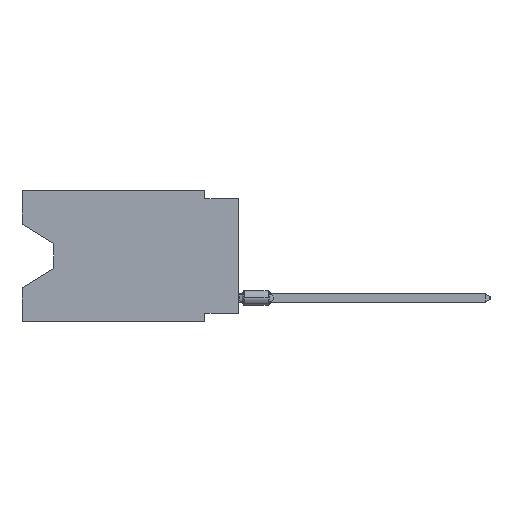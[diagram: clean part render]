
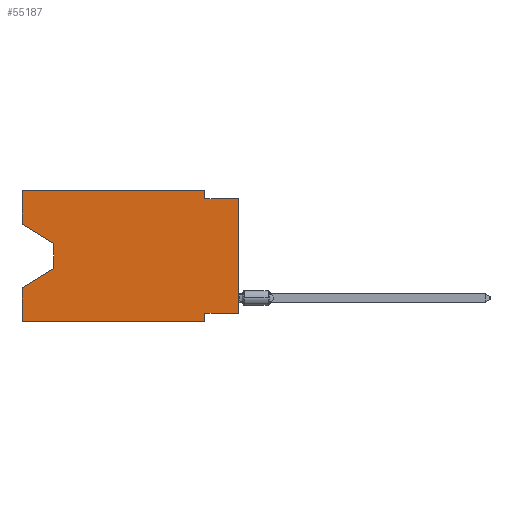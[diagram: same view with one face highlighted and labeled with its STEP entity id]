
A CAD part, left-side view. The second image highlights one B-rep face of the part: STEP entity #55187.
In plain terms, the highlighted planar face has unit normal (-1, 0, 0).
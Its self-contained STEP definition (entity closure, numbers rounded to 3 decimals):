
#244 = LINE ( 'NONE', #58147, #23302 ) ;
#911 = VERTEX_POINT ( 'NONE', #13001 ) ;
#1676 = EDGE_CURVE ( 'NONE', #24414, #61593, #34540, .T. ) ;
#2221 = DIRECTION ( 'NONE',  ( 0., -1., 0. ) ) ;
#2526 = VECTOR ( 'NONE', #54785, 1000. ) ;
#3853 = VECTOR ( 'NONE', #38729, 1000. ) ;
#5923 = CARTESIAN_POINT ( 'NONE',  ( 0., 16.383, 0. ) ) ;
#5988 = LINE ( 'NONE', #9868, #21817 ) ;
#6323 = DIRECTION ( 'NONE',  ( 0., 0., -1. ) ) ;
#6400 = AXIS2_PLACEMENT_3D ( 'NONE', #39036, #55075, #6996 ) ;
#6870 = CARTESIAN_POINT ( 'NONE',  ( 0., 0., -0.635 ) ) ;
#6996 = DIRECTION ( 'NONE',  ( 0., 0., -1. ) ) ;
#7610 = CARTESIAN_POINT ( 'NONE',  ( 0., 2.54, -9.271 ) ) ;
#7929 = CARTESIAN_POINT ( 'NONE',  ( 0., 16.383, -7.36 ) ) ;
#8169 = CARTESIAN_POINT ( 'NONE',  ( 0., 0., -0.635 ) ) ;
#9366 = ORIENTED_EDGE ( 'NONE', *, *, #19558, .F. ) ;
#9517 = VECTOR ( 'NONE', #2221, 1000. ) ;
#9868 = CARTESIAN_POINT ( 'NONE',  ( 0., 2.54, -9.906 ) ) ;
#10898 = VERTEX_POINT ( 'NONE', #7929 ) ;
#11689 = VERTEX_POINT ( 'NONE', #51573 ) ;
#12729 = VECTOR ( 'NONE', #14229, 1000. ) ;
#13001 = CARTESIAN_POINT ( 'NONE',  ( 0., 2.54, -9.906 ) ) ;
#13111 = CARTESIAN_POINT ( 'NONE',  ( 0., 0., -9.271 ) ) ;
#13189 = LINE ( 'NONE', #13889, #12729 ) ;
#13889 = CARTESIAN_POINT ( 'NONE',  ( 0., 16.383, 0. ) ) ;
#14229 = DIRECTION ( 'NONE',  ( 0., 0., 1. ) ) ;
#14278 = VECTOR ( 'NONE', #56601, 1000. ) ;
#15689 = DIRECTION ( 'NONE',  ( 0., -1., 0. ) ) ;
#16171 = VERTEX_POINT ( 'NONE', #47012 ) ;
#18167 = CARTESIAN_POINT ( 'NONE',  ( 0., 16.383, 0. ) ) ;
#19558 = EDGE_CURVE ( 'NONE', #32609, #10898, #38389, .T. ) ;
#19913 = ORIENTED_EDGE ( 'NONE', *, *, #37666, .T. ) ;
#20381 = EDGE_CURVE ( 'NONE', #32609, #911, #60815, .T. ) ;
#21331 = DIRECTION ( 'NONE',  ( 0., -0.855, -0.519 ) ) ;
#21817 = VECTOR ( 'NONE', #31117, 1000. ) ;
#22386 = LINE ( 'NONE', #64577, #2526 ) ;
#22391 = CARTESIAN_POINT ( 'NONE',  ( 0., 13.97, -4.013 ) ) ;
#23302 = VECTOR ( 'NONE', #53229, 1000. ) ;
#23369 = CARTESIAN_POINT ( 'NONE',  ( 0., 13.97, -5.893 ) ) ;
#24414 = VERTEX_POINT ( 'NONE', #49823 ) ;
#24623 = EDGE_CURVE ( 'NONE', #60272, #49423, #244, .T. ) ;
#24779 = DIRECTION ( 'NONE',  ( 0., 0., 1. ) ) ;
#27459 = ORIENTED_EDGE ( 'NONE', *, *, #1676, .F. ) ;
#27554 = FACE_OUTER_BOUND ( 'NONE', #32052, .T. ) ;
#28298 = VECTOR ( 'NONE', #15689, 1000. ) ;
#28327 = EDGE_CURVE ( 'NONE', #11689, #24414, #57886, .T. ) ;
#28705 = CARTESIAN_POINT ( 'NONE',  ( 0., 16.383, -9.906 ) ) ;
#29189 = VECTOR ( 'NONE', #21331, 1000. ) ;
#31117 = DIRECTION ( 'NONE',  ( 0., 0., -1. ) ) ;
#31757 = VERTEX_POINT ( 'NONE', #6870 ) ;
#32052 = EDGE_LOOP ( 'NONE', ( #51289, #41936, #38336, #9366, #62065, #38538, #60744, #19913, #34408, #27459, #47963, #59722 ) ) ;
#32609 = VERTEX_POINT ( 'NONE', #28705 ) ;
#32967 = EDGE_CURVE ( 'NONE', #49884, #911, #5988, .T. ) ;
#34408 = ORIENTED_EDGE ( 'NONE', *, *, #42374, .F. ) ;
#34540 = LINE ( 'NONE', #54399, #65931 ) ;
#37359 = LINE ( 'NONE', #37703, #29189 ) ;
#37666 = EDGE_CURVE ( 'NONE', #59210, #31757, #51957, .T. ) ;
#37703 = CARTESIAN_POINT ( 'NONE',  ( 0., 16.383, -2.546 ) ) ;
#38336 = ORIENTED_EDGE ( 'NONE', *, *, #62720, .T. ) ;
#38389 = LINE ( 'NONE', #18167, #3853 ) ;
#38538 = ORIENTED_EDGE ( 'NONE', *, *, #32967, .F. ) ;
#38729 = DIRECTION ( 'NONE',  ( 0., 0., 1. ) ) ;
#39036 = CARTESIAN_POINT ( 'NONE',  ( 0., 16.383, 0. ) ) ;
#40620 = EDGE_CURVE ( 'NONE', #59210, #49884, #65741, .T. ) ;
#41936 = ORIENTED_EDGE ( 'NONE', *, *, #24623, .T. ) ;
#42374 = EDGE_CURVE ( 'NONE', #61593, #31757, #61506, .T. ) ;
#43424 = DIRECTION ( 'NONE',  ( 0., 1., 0. ) ) ;
#45515 = VECTOR ( 'NONE', #24779, 1000. ) ;
#47012 = CARTESIAN_POINT ( 'NONE',  ( 0., 16.383, -2.546 ) ) ;
#47412 = EDGE_CURVE ( 'NONE', #16171, #60272, #37359, .T. ) ;
#47963 = ORIENTED_EDGE ( 'NONE', *, *, #28327, .F. ) ;
#48800 = PLANE ( 'NONE',  #6400 ) ;
#49017 = CARTESIAN_POINT ( 'NONE',  ( 0., 0., -9.271 ) ) ;
#49423 = VERTEX_POINT ( 'NONE', #23369 ) ;
#49624 = CARTESIAN_POINT ( 'NONE',  ( 0., 16.383, -9.906 ) ) ;
#49823 = CARTESIAN_POINT ( 'NONE',  ( 0., 2.54, 0. ) ) ;
#49884 = VERTEX_POINT ( 'NONE', #7610 ) ;
#51289 = ORIENTED_EDGE ( 'NONE', *, *, #47412, .T. ) ;
#51573 = CARTESIAN_POINT ( 'NONE',  ( 0., 16.383, 0. ) ) ;
#51607 = CARTESIAN_POINT ( 'NONE',  ( 0., 0., 0. ) ) ;
#51700 = EDGE_CURVE ( 'NONE', #16171, #11689, #13189, .T. ) ;
#51957 = LINE ( 'NONE', #51607, #45515 ) ;
#53229 = DIRECTION ( 'NONE',  ( 0., 0., -1. ) ) ;
#54399 = CARTESIAN_POINT ( 'NONE',  ( 0., 2.54, 0. ) ) ;
#54785 = DIRECTION ( 'NONE',  ( 0., 0.855, -0.519 ) ) ;
#55075 = DIRECTION ( 'NONE',  ( 1., 0., 0. ) ) ;
#55187 = ADVANCED_FACE ( 'NONE', ( #27554 ), #48800, .F. ) ;
#56601 = DIRECTION ( 'NONE',  ( 0., -1., 0. ) ) ;
#57886 = LINE ( 'NONE', #5923, #28298 ) ;
#58147 = CARTESIAN_POINT ( 'NONE',  ( 0., 13.97, -4.013 ) ) ;
#59210 = VERTEX_POINT ( 'NONE', #49017 ) ;
#59722 = ORIENTED_EDGE ( 'NONE', *, *, #51700, .F. ) ;
#60272 = VERTEX_POINT ( 'NONE', #22391 ) ;
#60744 = ORIENTED_EDGE ( 'NONE', *, *, #40620, .F. ) ;
#60815 = LINE ( 'NONE', #49624, #9517 ) ;
#61506 = LINE ( 'NONE', #8169, #14278 ) ;
#61593 = VERTEX_POINT ( 'NONE', #63962 ) ;
#62065 = ORIENTED_EDGE ( 'NONE', *, *, #20381, .T. ) ;
#62720 = EDGE_CURVE ( 'NONE', #49423, #10898, #22386, .T. ) ;
#63962 = CARTESIAN_POINT ( 'NONE',  ( 0., 2.54, -0.635 ) ) ;
#64577 = CARTESIAN_POINT ( 'NONE',  ( 0., 13.97, -5.893 ) ) ;
#65741 = LINE ( 'NONE', #13111, #68652 ) ;
#65931 = VECTOR ( 'NONE', #6323, 1000. ) ;
#68652 = VECTOR ( 'NONE', #43424, 1000. ) ;
